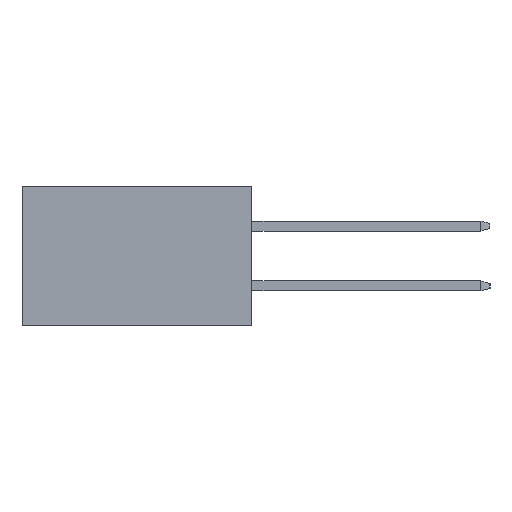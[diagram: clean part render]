
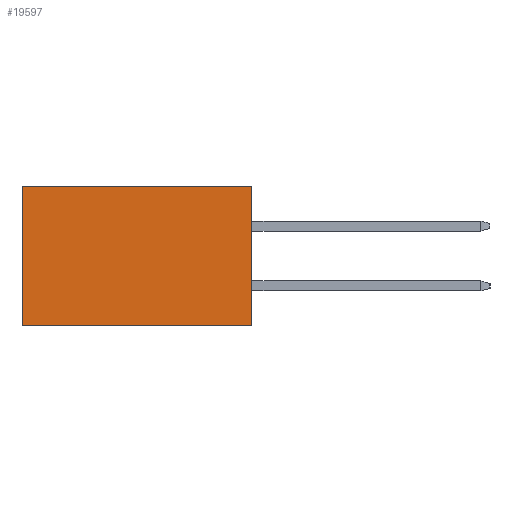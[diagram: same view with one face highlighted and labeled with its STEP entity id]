
A CAD part, left-side view. The second image highlights one B-rep face of the part: STEP entity #19597.
In plain terms, the highlighted planar face has unit normal (-1, 0, 0).
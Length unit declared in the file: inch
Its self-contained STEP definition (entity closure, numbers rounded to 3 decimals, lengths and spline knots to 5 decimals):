
#354 = VECTOR ( 'NONE', #8178, 39.37008 ) ;
#1884 = CARTESIAN_POINT ( 'NONE',  ( 0.3205, 0., -0.437 ) ) ;
#2280 = LINE ( 'NONE', #2472, #7430 ) ;
#2295 = LINE ( 'NONE', #9934, #10087 ) ;
#2322 = VERTEX_POINT ( 'NONE', #14491 ) ;
#2472 = CARTESIAN_POINT ( 'NONE',  ( 0.3205, 0.72, -0.437 ) ) ;
#2748 = PLANE ( 'NONE',  #11434 ) ;
#3627 = EDGE_CURVE ( 'NONE', #18513, #19362, #2280, .T. ) ;
#4501 = DIRECTION ( 'NONE',  ( 0., 0., -1. ) ) ;
#4878 = CARTESIAN_POINT ( 'NONE',  ( 0.3205, 0.72, -0.437 ) ) ;
#7430 = VECTOR ( 'NONE', #19534, 39.37008 ) ;
#7648 = DIRECTION ( 'NONE',  ( 0., 1., 0. ) ) ;
#8178 = DIRECTION ( 'NONE',  ( 0., 0., -1. ) ) ;
#8295 = EDGE_CURVE ( 'NONE', #8712, #2322, #16031, .T. ) ;
#8712 = VERTEX_POINT ( 'NONE', #17951 ) ;
#9934 = CARTESIAN_POINT ( 'NONE',  ( 0.3205, 0., 0. ) ) ;
#10025 = DIRECTION ( 'NONE',  ( 0., 1., 0. ) ) ;
#10087 = VECTOR ( 'NONE', #10025, 39.37008 ) ;
#10211 = EDGE_CURVE ( 'NONE', #8712, #18513, #2295, .T. ) ;
#10485 = EDGE_CURVE ( 'NONE', #2322, #19362, #18194, .T. ) ;
#11015 = FACE_OUTER_BOUND ( 'NONE', #14350, .T. ) ;
#11434 = AXIS2_PLACEMENT_3D ( 'NONE', #18660, #12361, #4501 ) ;
#12361 = DIRECTION ( 'NONE',  ( 1., 0., 0. ) ) ;
#12443 = VECTOR ( 'NONE', #7648, 39.37008 ) ;
#14350 = EDGE_LOOP ( 'NONE', ( #17774, #16598, #16636, #16581 ) ) ;
#14491 = CARTESIAN_POINT ( 'NONE',  ( 0.3205, 0., -0.437 ) ) ;
#16031 = LINE ( 'NONE', #1884, #354 ) ;
#16581 = ORIENTED_EDGE ( 'NONE', *, *, #10211, .T. ) ;
#16598 = ORIENTED_EDGE ( 'NONE', *, *, #10485, .F. ) ;
#16636 = ORIENTED_EDGE ( 'NONE', *, *, #8295, .F. ) ;
#16650 = CARTESIAN_POINT ( 'NONE',  ( 0.3205, 0., -0.437 ) ) ;
#17774 = ORIENTED_EDGE ( 'NONE', *, *, #3627, .T. ) ;
#17951 = CARTESIAN_POINT ( 'NONE',  ( 0.3205, 0., 0. ) ) ;
#18144 = CARTESIAN_POINT ( 'NONE',  ( 0.3205, 0.72, 0. ) ) ;
#18194 = LINE ( 'NONE', #16650, #12443 ) ;
#18513 = VERTEX_POINT ( 'NONE', #18144 ) ;
#18660 = CARTESIAN_POINT ( 'NONE',  ( 0.3205, 0., -0.437 ) ) ;
#19362 = VERTEX_POINT ( 'NONE', #4878 ) ;
#19534 = DIRECTION ( 'NONE',  ( 0., 0., -1. ) ) ;
#19597 = ADVANCED_FACE ( 'NONE', ( #11015 ), #2748, .F. ) ;
